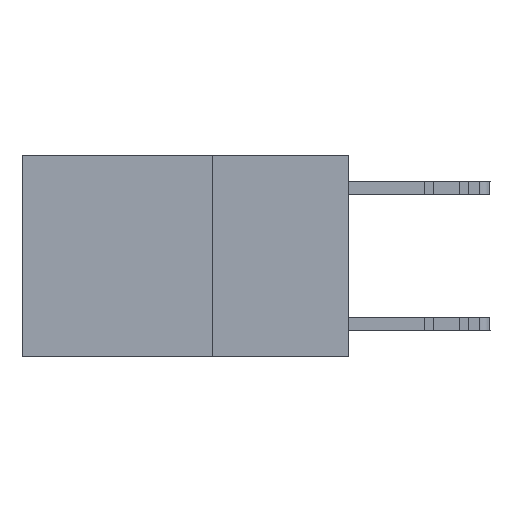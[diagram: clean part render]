
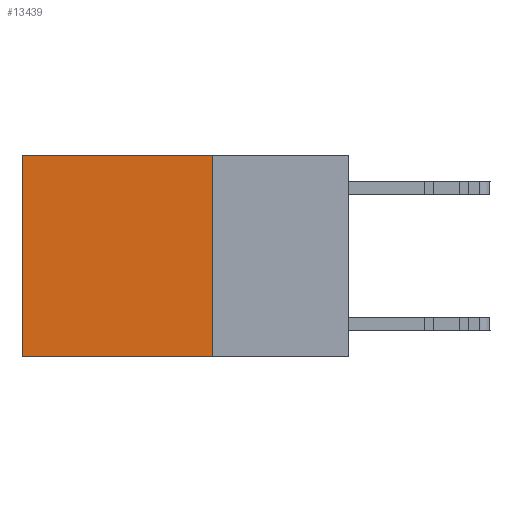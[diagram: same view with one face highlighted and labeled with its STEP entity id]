
A CAD part, left-side view. The second image highlights one B-rep face of the part: STEP entity #13439.
In plain terms, the highlighted planar face has unit normal (-1, 0, 0).
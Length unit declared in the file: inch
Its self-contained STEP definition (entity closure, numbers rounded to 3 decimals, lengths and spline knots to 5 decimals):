
#754 = CARTESIAN_POINT ( 'NONE',  ( 0.2625, 0.6, 0. ) ) ;
#1156 = EDGE_CURVE ( 'NONE', #11337, #10081, #21000, .T. ) ;
#2188 = CARTESIAN_POINT ( 'NONE',  ( 0.2625, 0.6, 0. ) ) ;
#4470 = CARTESIAN_POINT ( 'NONE',  ( 0.2625, 0.25, 0. ) ) ;
#4901 = LINE ( 'NONE', #14203, #20650 ) ;
#5858 = ORIENTED_EDGE ( 'NONE', *, *, #1156, .T. ) ;
#6811 = VERTEX_POINT ( 'NONE', #20484 ) ;
#7081 = PLANE ( 'NONE',  #11123 ) ;
#7235 = DIRECTION ( 'NONE',  ( 0., 0., -1. ) ) ;
#8841 = VERTEX_POINT ( 'NONE', #28646 ) ;
#9231 = ORIENTED_EDGE ( 'NONE', *, *, #9378, .F. ) ;
#9378 = EDGE_CURVE ( 'NONE', #11337, #8841, #18485, .T. ) ;
#9615 = CARTESIAN_POINT ( 'NONE',  ( 0.2625, 0.25, 0. ) ) ;
#9815 = CARTESIAN_POINT ( 'NONE',  ( 0.2625, 0.25, 0. ) ) ;
#10081 = VERTEX_POINT ( 'NONE', #754 ) ;
#11123 = AXIS2_PLACEMENT_3D ( 'NONE', #9815, #14545, #7235 ) ;
#11337 = VERTEX_POINT ( 'NONE', #4470 ) ;
#11492 = CARTESIAN_POINT ( 'NONE',  ( 0.2625, 0.25, 0. ) ) ;
#13179 = ORIENTED_EDGE ( 'NONE', *, *, #25377, .F. ) ;
#13439 = ADVANCED_FACE ( 'NONE', ( #20917 ), #7081, .F. ) ;
#14203 = CARTESIAN_POINT ( 'NONE',  ( 0.2625, 0.25, -0.37 ) ) ;
#14545 = DIRECTION ( 'NONE',  ( 1., 0., 0. ) ) ;
#14588 = EDGE_LOOP ( 'NONE', ( #24978, #13179, #9231, #5858 ) ) ;
#16345 = DIRECTION ( 'NONE',  ( 0., 1., 0. ) ) ;
#16466 = DIRECTION ( 'NONE',  ( 0., 1., 0. ) ) ;
#18485 = LINE ( 'NONE', #11492, #21233 ) ;
#18491 = LINE ( 'NONE', #2188, #25932 ) ;
#20484 = CARTESIAN_POINT ( 'NONE',  ( 0.2625, 0.6, -0.37 ) ) ;
#20650 = VECTOR ( 'NONE', #16345, 39.37008 ) ;
#20762 = DIRECTION ( 'NONE',  ( 0., 0., -1. ) ) ;
#20917 = FACE_OUTER_BOUND ( 'NONE', #14588, .T. ) ;
#21000 = LINE ( 'NONE', #9615, #22119 ) ;
#21233 = VECTOR ( 'NONE', #25639, 39.37008 ) ;
#22119 = VECTOR ( 'NONE', #16466, 39.37008 ) ;
#23616 = EDGE_CURVE ( 'NONE', #10081, #6811, #18491, .T. ) ;
#24978 = ORIENTED_EDGE ( 'NONE', *, *, #23616, .T. ) ;
#25377 = EDGE_CURVE ( 'NONE', #8841, #6811, #4901, .T. ) ;
#25639 = DIRECTION ( 'NONE',  ( 0., 0., -1. ) ) ;
#25932 = VECTOR ( 'NONE', #20762, 39.37008 ) ;
#28646 = CARTESIAN_POINT ( 'NONE',  ( 0.2625, 0.25, -0.37 ) ) ;
